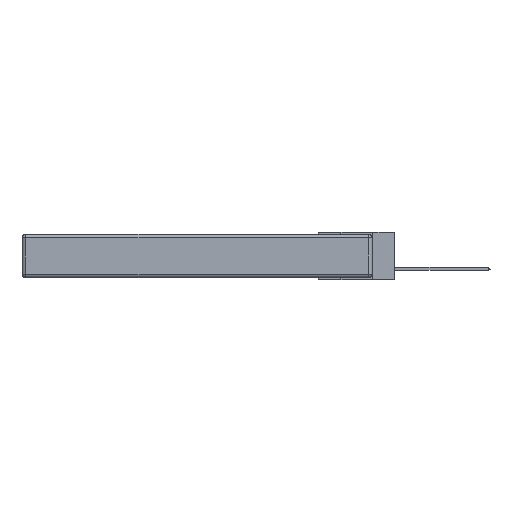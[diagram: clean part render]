
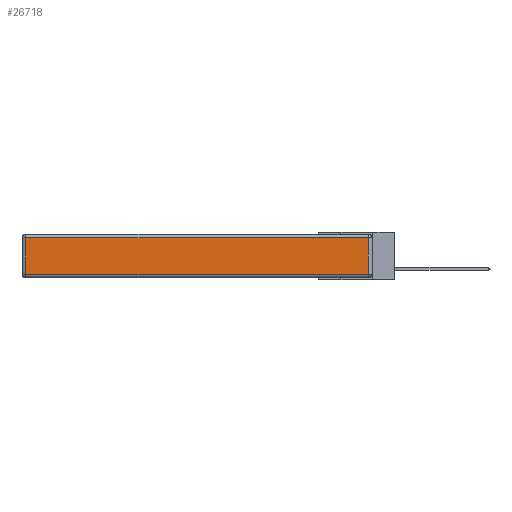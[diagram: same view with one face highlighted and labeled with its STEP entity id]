
A CAD part, left-side view. The second image highlights one B-rep face of the part: STEP entity #26718.
In plain terms, the highlighted planar face has unit normal (-1, 0, 0).
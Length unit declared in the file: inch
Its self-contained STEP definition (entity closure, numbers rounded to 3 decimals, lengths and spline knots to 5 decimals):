
#632 = VECTOR ( 'NONE', #15993, 39.37008 ) ;
#3624 = VECTOR ( 'NONE', #26524, 39.37008 ) ;
#3872 = ORIENTED_EDGE ( 'NONE', *, *, #30371, .T. ) ;
#4069 = ORIENTED_EDGE ( 'NONE', *, *, #12801, .T. ) ;
#5471 = AXIS2_PLACEMENT_3D ( 'NONE', #29162, #24381, #6705 ) ;
#5475 = VERTEX_POINT ( 'NONE', #8099 ) ;
#5500 = EDGE_LOOP ( 'NONE', ( #26427, #4069, #32109, #3872 ) ) ;
#6296 = FACE_OUTER_BOUND ( 'NONE', #5500, .T. ) ;
#6705 = DIRECTION ( 'NONE',  ( 0., 0., 1. ) ) ;
#8099 = CARTESIAN_POINT ( 'NONE',  ( 0., 0.03, -0.313 ) ) ;
#10218 = LINE ( 'NONE', #16916, #3624 ) ;
#10854 = CARTESIAN_POINT ( 'NONE',  ( 0., 0.03, -0.03 ) ) ;
#11071 = CARTESIAN_POINT ( 'NONE',  ( 0., 2.72, -0.343 ) ) ;
#12801 = EDGE_CURVE ( 'NONE', #5475, #25324, #22801, .T. ) ;
#13451 = VECTOR ( 'NONE', #21165, 39.37008 ) ;
#15280 = VERTEX_POINT ( 'NONE', #16481 ) ;
#15427 = VECTOR ( 'NONE', #29889, 39.37008 ) ;
#15993 = DIRECTION ( 'NONE',  ( 0., 0., -1. ) ) ;
#16184 = CARTESIAN_POINT ( 'NONE',  ( 0., 0., -0.313 ) ) ;
#16481 = CARTESIAN_POINT ( 'NONE',  ( 0., 2.72, -0.313 ) ) ;
#16916 = CARTESIAN_POINT ( 'NONE',  ( 0., 2.75, -0.03 ) ) ;
#19608 = CARTESIAN_POINT ( 'NONE',  ( 0., 2.72, -0.03 ) ) ;
#19869 = CARTESIAN_POINT ( 'NONE',  ( 0., 0.03, -0.343 ) ) ;
#20246 = EDGE_CURVE ( 'NONE', #25324, #22714, #10218, .T. ) ;
#21165 = DIRECTION ( 'NONE',  ( 0., -1., 0. ) ) ;
#22714 = VERTEX_POINT ( 'NONE', #19608 ) ;
#22801 = LINE ( 'NONE', #19869, #15427 ) ;
#24381 = DIRECTION ( 'NONE',  ( -1., 0., 0. ) ) ;
#25310 = EDGE_CURVE ( 'NONE', #15280, #5475, #27483, .T. ) ;
#25324 = VERTEX_POINT ( 'NONE', #10854 ) ;
#26427 = ORIENTED_EDGE ( 'NONE', *, *, #25310, .T. ) ;
#26524 = DIRECTION ( 'NONE',  ( 0., 1., 0. ) ) ;
#26718 = ADVANCED_FACE ( 'NONE', ( #6296 ), #29268, .T. ) ;
#27483 = LINE ( 'NONE', #16184, #13451 ) ;
#29162 = CARTESIAN_POINT ( 'NONE',  ( 0., 0., -0.343 ) ) ;
#29268 = PLANE ( 'NONE',  #5471 ) ;
#29467 = LINE ( 'NONE', #11071, #632 ) ;
#29889 = DIRECTION ( 'NONE',  ( 0., 0., 1. ) ) ;
#30371 = EDGE_CURVE ( 'NONE', #22714, #15280, #29467, .T. ) ;
#32109 = ORIENTED_EDGE ( 'NONE', *, *, #20246, .T. ) ;
